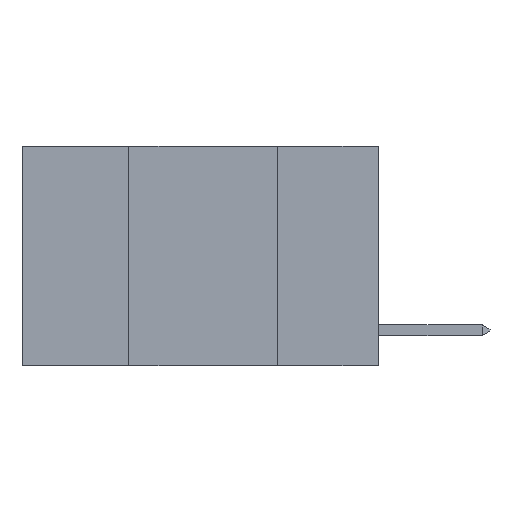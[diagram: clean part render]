
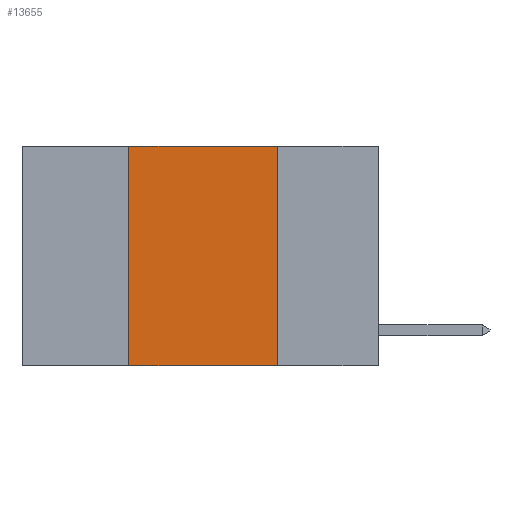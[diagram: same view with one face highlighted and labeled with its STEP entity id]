
A CAD part, left-side view. The second image highlights one B-rep face of the part: STEP entity #13655.
In plain terms, the highlighted planar face has unit normal (-1, 0, 0).
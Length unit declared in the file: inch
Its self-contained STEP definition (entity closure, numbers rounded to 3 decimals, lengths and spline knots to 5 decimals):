
#240 = CARTESIAN_POINT ( 'NONE',  ( 0., 0.17, 0. ) ) ;
#746 = DIRECTION ( 'NONE',  ( 0., -1., 0. ) ) ;
#761 = AXIS2_PLACEMENT_3D ( 'NONE', #14154, #14381, #6386 ) ;
#776 = EDGE_CURVE ( 'NONE', #5013, #12888, #10767, .T. ) ;
#1002 = FACE_OUTER_BOUND ( 'NONE', #4398, .T. ) ;
#1096 = CARTESIAN_POINT ( 'NONE',  ( 0., 0.42, 0. ) ) ;
#2321 = VECTOR ( 'NONE', #10898, 39.37008 ) ;
#2590 = EDGE_CURVE ( 'NONE', #5013, #16449, #12635, .T. ) ;
#2939 = CARTESIAN_POINT ( 'NONE',  ( 0., 0.17, -0.37 ) ) ;
#3103 = VERTEX_POINT ( 'NONE', #5071 ) ;
#4171 = CARTESIAN_POINT ( 'NONE',  ( 0., 0.6, 0. ) ) ;
#4398 = EDGE_LOOP ( 'NONE', ( #11465, #16521, #10201, #14570 ) ) ;
#4895 = DIRECTION ( 'NONE',  ( 0., 0., 1. ) ) ;
#5013 = VERTEX_POINT ( 'NONE', #15898 ) ;
#5071 = CARTESIAN_POINT ( 'NONE',  ( 0., 0.17, 0. ) ) ;
#5247 = VECTOR ( 'NONE', #13517, 39.37008 ) ;
#6386 = DIRECTION ( 'NONE',  ( 0., 0., -1. ) ) ;
#7483 = CARTESIAN_POINT ( 'NONE',  ( 0., 0.6, -0.37 ) ) ;
#7861 = EDGE_CURVE ( 'NONE', #3103, #12888, #12986, .T. ) ;
#8008 = CARTESIAN_POINT ( 'NONE',  ( 0., 0.42, 0. ) ) ;
#9957 = VECTOR ( 'NONE', #746, 39.37008 ) ;
#10201 = ORIENTED_EDGE ( 'NONE', *, *, #2590, .F. ) ;
#10767 = LINE ( 'NONE', #7483, #9957 ) ;
#10898 = DIRECTION ( 'NONE',  ( 0., -1., 0. ) ) ;
#11465 = ORIENTED_EDGE ( 'NONE', *, *, #7861, .F. ) ;
#12552 = EDGE_CURVE ( 'NONE', #16449, #3103, #16520, .T. ) ;
#12635 = LINE ( 'NONE', #8008, #16407 ) ;
#12888 = VERTEX_POINT ( 'NONE', #2939 ) ;
#12986 = LINE ( 'NONE', #240, #5247 ) ;
#13517 = DIRECTION ( 'NONE',  ( 0., 0., -1. ) ) ;
#13655 = ADVANCED_FACE ( 'NONE', ( #1002 ), #15635, .F. ) ;
#14154 = CARTESIAN_POINT ( 'NONE',  ( 0., 0.6, 0. ) ) ;
#14381 = DIRECTION ( 'NONE',  ( 1., 0., 0. ) ) ;
#14570 = ORIENTED_EDGE ( 'NONE', *, *, #776, .T. ) ;
#15635 = PLANE ( 'NONE',  #761 ) ;
#15898 = CARTESIAN_POINT ( 'NONE',  ( 0., 0.42, -0.37 ) ) ;
#16407 = VECTOR ( 'NONE', #4895, 39.37008 ) ;
#16449 = VERTEX_POINT ( 'NONE', #1096 ) ;
#16520 = LINE ( 'NONE', #4171, #2321 ) ;
#16521 = ORIENTED_EDGE ( 'NONE', *, *, #12552, .F. ) ;
